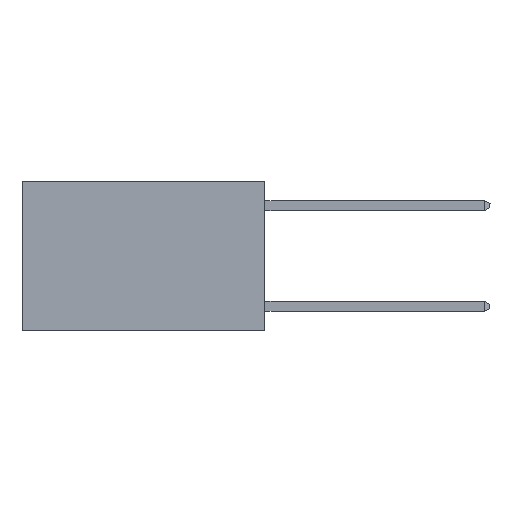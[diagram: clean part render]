
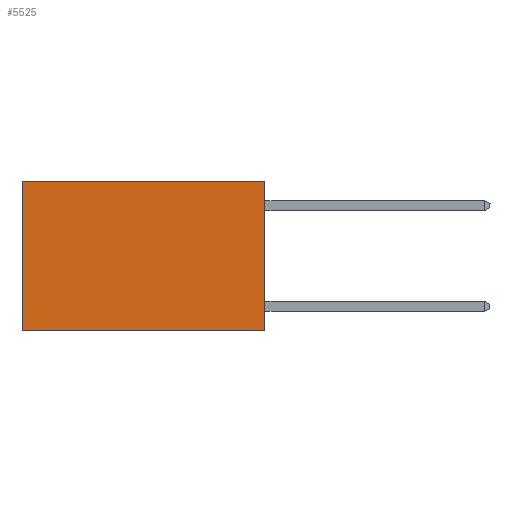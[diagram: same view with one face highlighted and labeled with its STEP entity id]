
A CAD part, left-side view. The second image highlights one B-rep face of the part: STEP entity #5525.
In plain terms, the highlighted planar face has unit normal (-1, 0, 0).
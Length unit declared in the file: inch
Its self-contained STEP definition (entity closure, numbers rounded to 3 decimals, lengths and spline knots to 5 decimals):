
#955 = CARTESIAN_POINT ( 'NONE',  ( 0.2625, 0., -0.37 ) ) ;
#2167 = FACE_OUTER_BOUND ( 'NONE', #16455, .T. ) ;
#2253 = LINE ( 'NONE', #17379, #16302 ) ;
#2349 = DIRECTION ( 'NONE',  ( 0., 0., -1. ) ) ;
#2953 = EDGE_CURVE ( 'NONE', #3748, #17811, #2253, .T. ) ;
#3748 = VERTEX_POINT ( 'NONE', #6905 ) ;
#4416 = ORIENTED_EDGE ( 'NONE', *, *, #10713, .T. ) ;
#5185 = DIRECTION ( 'NONE',  ( 0., 0., -1. ) ) ;
#5525 = ADVANCED_FACE ( 'NONE', ( #2167 ), #10541, .F. ) ;
#6274 = LINE ( 'NONE', #7989, #11910 ) ;
#6466 = ORIENTED_EDGE ( 'NONE', *, *, #2953, .T. ) ;
#6905 = CARTESIAN_POINT ( 'NONE',  ( 0.2625, 0., 0. ) ) ;
#7753 = DIRECTION ( 'NONE',  ( 0., 1., 0. ) ) ;
#7880 = DIRECTION ( 'NONE',  ( 1., 0., 0. ) ) ;
#7989 = CARTESIAN_POINT ( 'NONE',  ( 0.2625, 0., 0. ) ) ;
#8025 = LINE ( 'NONE', #10336, #9857 ) ;
#9266 = EDGE_CURVE ( 'NONE', #10201, #14606, #13545, .T. ) ;
#9499 = DIRECTION ( 'NONE',  ( 0., 0., -1. ) ) ;
#9857 = VECTOR ( 'NONE', #9499, 39.37008 ) ;
#10201 = VERTEX_POINT ( 'NONE', #15873 ) ;
#10336 = CARTESIAN_POINT ( 'NONE',  ( 0.2625, 0.6, 0. ) ) ;
#10534 = CARTESIAN_POINT ( 'NONE',  ( 0.2625, 0.6, 0. ) ) ;
#10541 = PLANE ( 'NONE',  #15514 ) ;
#10713 = EDGE_CURVE ( 'NONE', #17811, #14606, #8025, .T. ) ;
#11491 = EDGE_CURVE ( 'NONE', #3748, #10201, #6274, .T. ) ;
#11910 = VECTOR ( 'NONE', #5185, 39.37008 ) ;
#13146 = CARTESIAN_POINT ( 'NONE',  ( 0.2625, 0., 0. ) ) ;
#13152 = ORIENTED_EDGE ( 'NONE', *, *, #11491, .F. ) ;
#13545 = LINE ( 'NONE', #955, #16451 ) ;
#13793 = CARTESIAN_POINT ( 'NONE',  ( 0.2625, 0.6, -0.37 ) ) ;
#14606 = VERTEX_POINT ( 'NONE', #13793 ) ;
#15097 = ORIENTED_EDGE ( 'NONE', *, *, #9266, .F. ) ;
#15514 = AXIS2_PLACEMENT_3D ( 'NONE', #13146, #7880, #2349 ) ;
#15873 = CARTESIAN_POINT ( 'NONE',  ( 0.2625, 0., -0.37 ) ) ;
#16302 = VECTOR ( 'NONE', #17194, 39.37008 ) ;
#16451 = VECTOR ( 'NONE', #7753, 39.37008 ) ;
#16455 = EDGE_LOOP ( 'NONE', ( #4416, #15097, #13152, #6466 ) ) ;
#17194 = DIRECTION ( 'NONE',  ( 0., 1., 0. ) ) ;
#17379 = CARTESIAN_POINT ( 'NONE',  ( 0.2625, 0., 0. ) ) ;
#17811 = VERTEX_POINT ( 'NONE', #10534 ) ;
